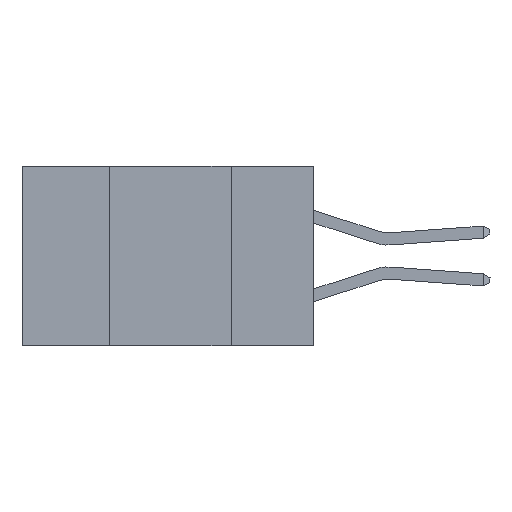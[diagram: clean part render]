
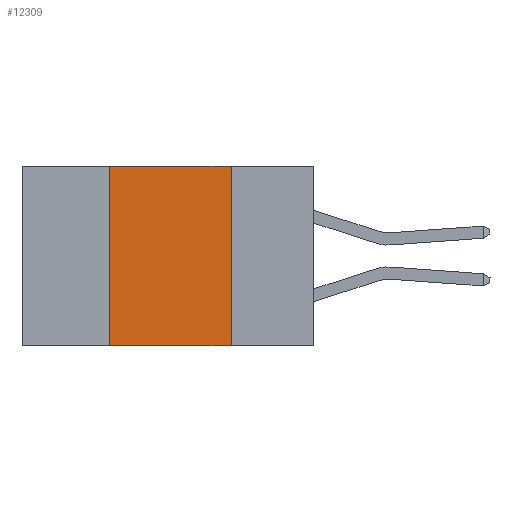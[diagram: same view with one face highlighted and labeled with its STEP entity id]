
A CAD part, left-side view. The second image highlights one B-rep face of the part: STEP entity #12309.
In plain terms, the highlighted planar face has unit normal (-1, 0, 0).
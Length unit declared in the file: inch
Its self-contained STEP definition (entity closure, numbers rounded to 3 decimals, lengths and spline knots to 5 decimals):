
#76 = PLANE ( 'NONE',  #17196 ) ;
#176 = VERTEX_POINT ( 'NONE', #20910 ) ;
#350 = CARTESIAN_POINT ( 'NONE',  ( 0., 0.42, -0.37 ) ) ;
#2052 = EDGE_CURVE ( 'NONE', #176, #21527, #20602, .T. ) ;
#2264 = EDGE_CURVE ( 'NONE', #17421, #7840, #21160, .T. ) ;
#2425 = VECTOR ( 'NONE', #12786, 39.37008 ) ;
#2759 = LINE ( 'NONE', #16949, #6725 ) ;
#4102 = CARTESIAN_POINT ( 'NONE',  ( 0., 0.17, -0.37 ) ) ;
#4203 = VECTOR ( 'NONE', #12393, 39.37008 ) ;
#4509 = ORIENTED_EDGE ( 'NONE', *, *, #18931, .F. ) ;
#4877 = FACE_OUTER_BOUND ( 'NONE', #15027, .T. ) ;
#5991 = CARTESIAN_POINT ( 'NONE',  ( 0., 0.6, 0. ) ) ;
#6682 = DIRECTION ( 'NONE',  ( 0., 0., -1. ) ) ;
#6725 = VECTOR ( 'NONE', #6682, 39.37008 ) ;
#6835 = LINE ( 'NONE', #15707, #4203 ) ;
#7317 = CARTESIAN_POINT ( 'NONE',  ( 0., 0.17, 0. ) ) ;
#7840 = VERTEX_POINT ( 'NONE', #4102 ) ;
#9794 = ORIENTED_EDGE ( 'NONE', *, *, #2264, .T. ) ;
#12309 = ADVANCED_FACE ( 'NONE', ( #4877 ), #76, .F. ) ;
#12393 = DIRECTION ( 'NONE',  ( 0., 0., 1. ) ) ;
#12786 = DIRECTION ( 'NONE',  ( 0., -1., 0. ) ) ;
#13265 = DIRECTION ( 'NONE',  ( 0., 0., -1. ) ) ;
#13514 = ORIENTED_EDGE ( 'NONE', *, *, #17640, .F. ) ;
#15027 = EDGE_LOOP ( 'NONE', ( #13514, #17317, #4509, #9794 ) ) ;
#15707 = CARTESIAN_POINT ( 'NONE',  ( 0., 0.42, 0. ) ) ;
#16949 = CARTESIAN_POINT ( 'NONE',  ( 0., 0.17, 0. ) ) ;
#16996 = CARTESIAN_POINT ( 'NONE',  ( 0., 0.6, -0.37 ) ) ;
#17196 = AXIS2_PLACEMENT_3D ( 'NONE', #21804, #18116, #13265 ) ;
#17317 = ORIENTED_EDGE ( 'NONE', *, *, #2052, .F. ) ;
#17421 = VERTEX_POINT ( 'NONE', #350 ) ;
#17640 = EDGE_CURVE ( 'NONE', #21527, #7840, #2759, .T. ) ;
#18116 = DIRECTION ( 'NONE',  ( 1., 0., 0. ) ) ;
#18931 = EDGE_CURVE ( 'NONE', #17421, #176, #6835, .T. ) ;
#20325 = VECTOR ( 'NONE', #22142, 39.37008 ) ;
#20602 = LINE ( 'NONE', #5991, #2425 ) ;
#20910 = CARTESIAN_POINT ( 'NONE',  ( 0., 0.42, 0. ) ) ;
#21160 = LINE ( 'NONE', #16996, #20325 ) ;
#21527 = VERTEX_POINT ( 'NONE', #7317 ) ;
#21804 = CARTESIAN_POINT ( 'NONE',  ( 0., 0.6, 0. ) ) ;
#22142 = DIRECTION ( 'NONE',  ( 0., -1., 0. ) ) ;
